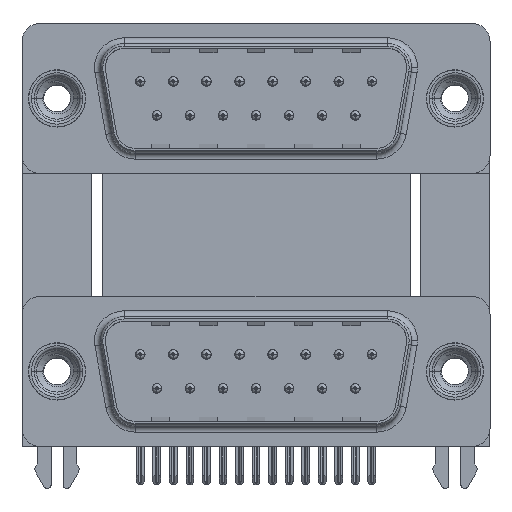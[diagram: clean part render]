
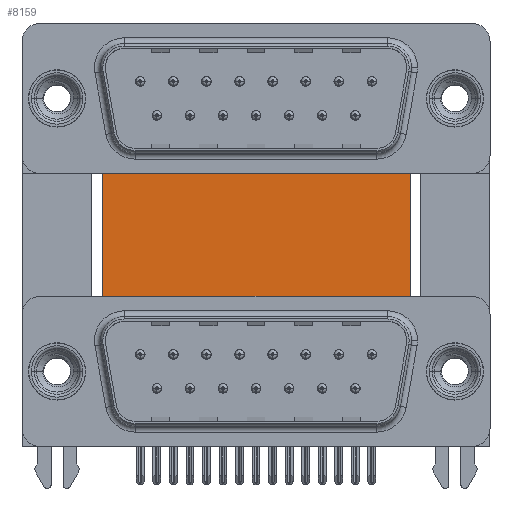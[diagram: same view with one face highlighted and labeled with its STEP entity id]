
A CAD part, top view. The second image highlights one B-rep face of the part: STEP entity #8159.
In plain terms, the highlighted planar face has unit normal (0, 0, 1).
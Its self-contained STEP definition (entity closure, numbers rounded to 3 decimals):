
#689 = LINE ( 'NONE', #10983, #4834 ) ;
#1063 = EDGE_CURVE ( 'NONE', #25255, #23483, #689, .T. ) ;
#1548 = VECTOR ( 'NONE', #7697, 1000. ) ;
#2177 = CARTESIAN_POINT ( 'NONE',  ( 3.79, 16.585, -12. ) ) ;
#2206 = LINE ( 'NONE', #22083, #32518 ) ;
#2426 = PLANE ( 'NONE',  #5867 ) ;
#2522 = CARTESIAN_POINT ( 'NONE',  ( 29.58, -3.735, -12. ) ) ;
#2639 = ORIENTED_EDGE ( 'NONE', *, *, #11053, .T. ) ;
#4834 = VECTOR ( 'NONE', #21234, 1000. ) ;
#4888 = DIRECTION ( 'NONE',  ( 1., 0., 0. ) ) ;
#5481 = DIRECTION ( 'NONE',  ( 0., 0., -1. ) ) ;
#5867 = AXIS2_PLACEMENT_3D ( 'NONE', #22982, #5481, #15731 ) ;
#6475 = EDGE_LOOP ( 'NONE', ( #31342, #16323, #32422, #2639 ) ) ;
#7239 = EDGE_CURVE ( 'NONE', #17597, #10009, #17673, .T. ) ;
#7697 = DIRECTION ( 'NONE',  ( 0., -1., 0. ) ) ;
#8159 = ADVANCED_FACE ( 'NONE', ( #18260 ), #2426, .F. ) ;
#10009 = VERTEX_POINT ( 'NONE', #11074 ) ;
#10983 = CARTESIAN_POINT ( 'NONE',  ( 3.79, -3.735, -12. ) ) ;
#11053 = EDGE_CURVE ( 'NONE', #17597, #25255, #22998, .T. ) ;
#11074 = CARTESIAN_POINT ( 'NONE',  ( 29.58, 16.585, -12. ) ) ;
#14336 = DIRECTION ( 'NONE',  ( 0., -1., 0. ) ) ;
#15731 = DIRECTION ( 'NONE',  ( -1., 0., 0. ) ) ;
#16323 = ORIENTED_EDGE ( 'NONE', *, *, #30515, .F. ) ;
#17597 = VERTEX_POINT ( 'NONE', #26159 ) ;
#17673 = LINE ( 'NONE', #2177, #18515 ) ;
#18260 = FACE_OUTER_BOUND ( 'NONE', #6475, .T. ) ;
#18515 = VECTOR ( 'NONE', #4888, 1000. ) ;
#20474 = CARTESIAN_POINT ( 'NONE',  ( 3.79, 16.585, -12. ) ) ;
#21234 = DIRECTION ( 'NONE',  ( 1., 0., 0. ) ) ;
#22083 = CARTESIAN_POINT ( 'NONE',  ( 29.58, 16.585, -12. ) ) ;
#22982 = CARTESIAN_POINT ( 'NONE',  ( 3.79, 16.585, -12. ) ) ;
#22998 = LINE ( 'NONE', #20474, #1548 ) ;
#23483 = VERTEX_POINT ( 'NONE', #2522 ) ;
#25255 = VERTEX_POINT ( 'NONE', #27200 ) ;
#26159 = CARTESIAN_POINT ( 'NONE',  ( 3.79, 16.585, -12. ) ) ;
#27200 = CARTESIAN_POINT ( 'NONE',  ( 3.79, -3.735, -12. ) ) ;
#30515 = EDGE_CURVE ( 'NONE', #10009, #23483, #2206, .T. ) ;
#31342 = ORIENTED_EDGE ( 'NONE', *, *, #1063, .T. ) ;
#32422 = ORIENTED_EDGE ( 'NONE', *, *, #7239, .F. ) ;
#32518 = VECTOR ( 'NONE', #14336, 1000. ) ;
